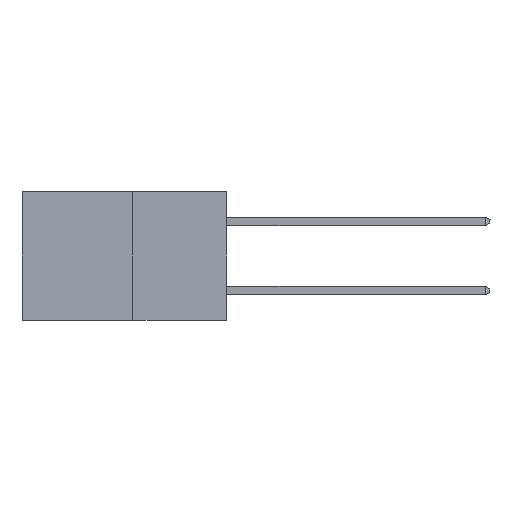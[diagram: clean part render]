
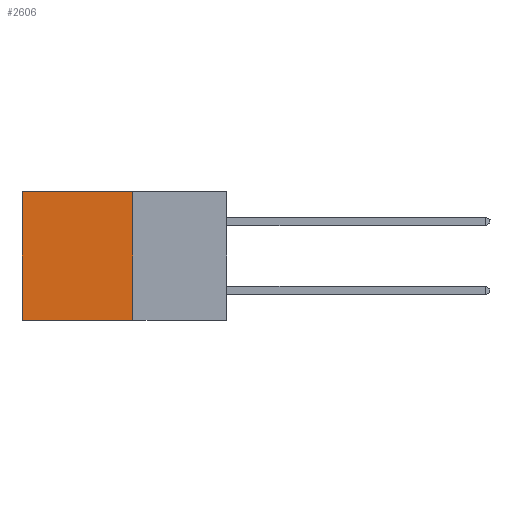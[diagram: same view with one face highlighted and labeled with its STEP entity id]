
A CAD part, left-side view. The second image highlights one B-rep face of the part: STEP entity #2606.
In plain terms, the highlighted planar face has unit normal (-1, 0, 0).
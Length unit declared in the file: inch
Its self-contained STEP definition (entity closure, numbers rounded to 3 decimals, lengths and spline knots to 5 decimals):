
#31 = DIRECTION ( 'NONE',  ( 0., 0., -1. ) ) ;
#112 = FACE_OUTER_BOUND ( 'NONE', #3359, .T. ) ;
#391 = LINE ( 'NONE', #4021, #5734 ) ;
#671 = EDGE_CURVE ( 'NONE', #6602, #2217, #5906, .T. ) ;
#1887 = EDGE_CURVE ( 'NONE', #8543, #6602, #7517, .T. ) ;
#1918 = ORIENTED_EDGE ( 'NONE', *, *, #8475, .T. ) ;
#2217 = VERTEX_POINT ( 'NONE', #7686 ) ;
#2262 = VECTOR ( 'NONE', #31, 39.37008 ) ;
#2282 = VECTOR ( 'NONE', #7674, 39.37008 ) ;
#2566 = PLANE ( 'NONE',  #2957 ) ;
#2606 = ADVANCED_FACE ( 'NONE', ( #112 ), #2566, .F. ) ;
#2957 = AXIS2_PLACEMENT_3D ( 'NONE', #7416, #7369, #4307 ) ;
#2965 = CARTESIAN_POINT ( 'NONE',  ( 0.277, 0.27, 0. ) ) ;
#3359 = EDGE_LOOP ( 'NONE', ( #1918, #5299, #8119, #4426 ) ) ;
#3810 = VECTOR ( 'NONE', #5182, 39.37008 ) ;
#3941 = DIRECTION ( 'NONE',  ( 0., 1., 0. ) ) ;
#4021 = CARTESIAN_POINT ( 'NONE',  ( 0.277, 0.27, 0. ) ) ;
#4307 = DIRECTION ( 'NONE',  ( 0., 0., -1. ) ) ;
#4426 = ORIENTED_EDGE ( 'NONE', *, *, #5593, .T. ) ;
#4893 = VERTEX_POINT ( 'NONE', #6767 ) ;
#5182 = DIRECTION ( 'NONE',  ( 0., 0., -1. ) ) ;
#5299 = ORIENTED_EDGE ( 'NONE', *, *, #671, .F. ) ;
#5593 = EDGE_CURVE ( 'NONE', #8543, #4893, #391, .T. ) ;
#5624 = CARTESIAN_POINT ( 'NONE',  ( 0.277, 0.27, -0.37 ) ) ;
#5734 = VECTOR ( 'NONE', #3941, 39.37008 ) ;
#5864 = CARTESIAN_POINT ( 'NONE',  ( 0.277, 0.27, -0.37 ) ) ;
#5906 = LINE ( 'NONE', #5624, #2282 ) ;
#6602 = VERTEX_POINT ( 'NONE', #5864 ) ;
#6767 = CARTESIAN_POINT ( 'NONE',  ( 0.277, 0.59, 0. ) ) ;
#7026 = LINE ( 'NONE', #8206, #2262 ) ;
#7369 = DIRECTION ( 'NONE',  ( 1., 0., 0. ) ) ;
#7416 = CARTESIAN_POINT ( 'NONE',  ( 0.277, 0.27, -0.37 ) ) ;
#7517 = LINE ( 'NONE', #8385, #3810 ) ;
#7674 = DIRECTION ( 'NONE',  ( 0., 1., 0. ) ) ;
#7686 = CARTESIAN_POINT ( 'NONE',  ( 0.277, 0.59, -0.37 ) ) ;
#8119 = ORIENTED_EDGE ( 'NONE', *, *, #1887, .F. ) ;
#8206 = CARTESIAN_POINT ( 'NONE',  ( 0.277, 0.59, -0.37 ) ) ;
#8385 = CARTESIAN_POINT ( 'NONE',  ( 0.277, 0.27, -0.37 ) ) ;
#8475 = EDGE_CURVE ( 'NONE', #4893, #2217, #7026, .T. ) ;
#8543 = VERTEX_POINT ( 'NONE', #2965 ) ;
